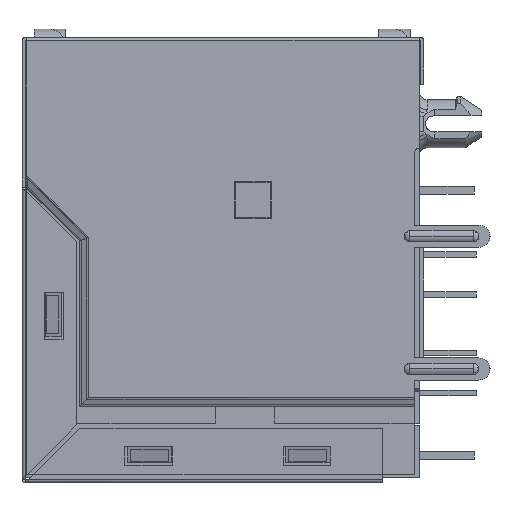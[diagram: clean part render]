
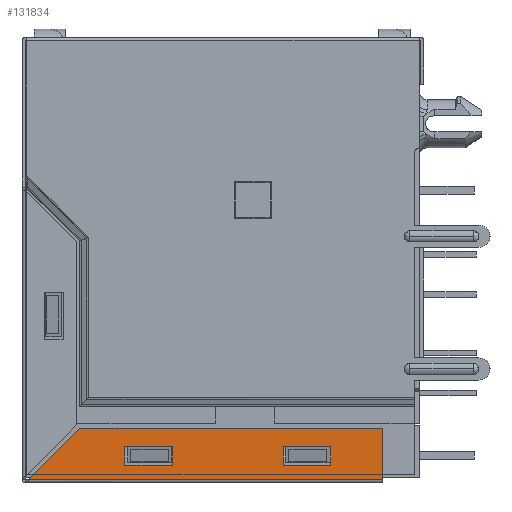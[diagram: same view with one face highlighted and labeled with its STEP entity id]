
A CAD part, left-side view. The second image highlights one B-rep face of the part: STEP entity #131834.
In plain terms, the highlighted planar face has unit normal (-1, 0, 0).
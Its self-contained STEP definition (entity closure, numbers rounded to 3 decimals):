
#479 = EDGE_CURVE ( 'NONE', #92332, #122461, #67862, .T. ) ;
#1755 = CARTESIAN_POINT ( 'NONE',  ( -31.875, -6.835, -26.78 ) ) ;
#2721 = CARTESIAN_POINT ( 'NONE',  ( -31.875, -6.835, -25.58 ) ) ;
#3954 = CARTESIAN_POINT ( 'NONE',  ( -31.875, 9.005, -24.43 ) ) ;
#6766 = CARTESIAN_POINT ( 'NONE',  ( -31.875, 9.005, -24.43 ) ) ;
#7658 = AXIS2_PLACEMENT_3D ( 'NONE', #82302, #104443, #136726 ) ;
#8901 = VERTEX_POINT ( 'NONE', #135240 ) ;
#9301 = ORIENTED_EDGE ( 'NONE', *, *, #128869, .T. ) ;
#12547 = VERTEX_POINT ( 'NONE', #30145 ) ;
#12951 = VERTEX_POINT ( 'NONE', #25709 ) ;
#13915 = EDGE_CURVE ( 'NONE', #138499, #12951, #78250, .T. ) ;
#15369 = CARTESIAN_POINT ( 'NONE',  ( -31.875, -6.835, -26.78 ) ) ;
#18320 = ORIENTED_EDGE ( 'NONE', *, *, #48286, .F. ) ;
#22806 = EDGE_CURVE ( 'NONE', #122461, #8901, #53511, .T. ) ;
#23165 = B_SPLINE_CURVE_WITH_KNOTS ( 'NONE', 1,
 ( #71344, #26937 ),
 .UNSPECIFIED., .F., .F.,
 ( 2, 2 ),
 ( 0., 1. ),
 .UNSPECIFIED. ) ;
#25709 = CARTESIAN_POINT ( 'NONE',  ( -31.875, -10.135, -24.43 ) ) ;
#26937 = CARTESIAN_POINT ( 'NONE',  ( -31.875, -10.135, -27.67 ) ) ;
#27816 = FACE_BOUND ( 'NONE', #97887, .T. ) ;
#28382 = EDGE_CURVE ( 'NONE', #57053, #57291, #94023, .T. ) ;
#30145 = CARTESIAN_POINT ( 'NONE',  ( -31.875, 3.165, -25.58 ) ) ;
#31083 = B_SPLINE_CURVE_WITH_KNOTS ( 'NONE', 1,
 ( #90847, #58183 ),
 .UNSPECIFIED., .F., .F.,
 ( 2, 2 ),
 ( 0., 1. ),
 .UNSPECIFIED. ) ;
#31956 = CARTESIAN_POINT ( 'NONE',  ( -31.875, -6.835, -25.58 ) ) ;
#37883 = CARTESIAN_POINT ( 'NONE',  ( -31.875, 12.245, -27.67 ) ) ;
#38693 = CARTESIAN_POINT ( 'NONE',  ( -31.875, 3.165, -26.78 ) ) ;
#43292 = CARTESIAN_POINT ( 'NONE',  ( -31.875, 3.165, -26.78 ) ) ;
#44898 = EDGE_CURVE ( 'NONE', #12547, #78756, #121286, .T. ) ;
#45583 = ORIENTED_EDGE ( 'NONE', *, *, #479, .T. ) ;
#47534 = CARTESIAN_POINT ( 'NONE',  ( -31.875, 3.165, -25.58 ) ) ;
#48286 = EDGE_CURVE ( 'NONE', #12951, #57291, #23165, .T. ) ;
#49384 = EDGE_LOOP ( 'NONE', ( #9301, #84357, #45583, #81935 ) ) ;
#51199 = CARTESIAN_POINT ( 'NONE',  ( -31.875, 12.245, -27.67 ) ) ;
#51403 = CARTESIAN_POINT ( 'NONE',  ( -31.875, -10.135, -24.43 ) ) ;
#53511 = B_SPLINE_CURVE_WITH_KNOTS ( 'NONE', 1,
 ( #82956, #61356 ),
 .UNSPECIFIED., .F., .F.,
 ( 2, 2 ),
 ( 0., 1. ),
 .UNSPECIFIED. ) ;
#53728 = CARTESIAN_POINT ( 'NONE',  ( -31.875, -3.835, -25.58 ) ) ;
#54936 = B_SPLINE_CURVE_WITH_KNOTS ( 'NONE', 1,
 ( #107171, #75411 ),
 .UNSPECIFIED., .F., .F.,
 ( 2, 2 ),
 ( 0., 1. ),
 .UNSPECIFIED. ) ;
#55385 = EDGE_LOOP ( 'NONE', ( #62046, #84402, #18320, #114992 ) ) ;
#56720 = CARTESIAN_POINT ( 'NONE',  ( -31.875, 6.165, -26.78 ) ) ;
#57053 = VERTEX_POINT ( 'NONE', #51199 ) ;
#57291 = VERTEX_POINT ( 'NONE', #133423 ) ;
#58183 = CARTESIAN_POINT ( 'NONE',  ( -31.875, 6.165, -25.58 ) ) ;
#60701 = EDGE_CURVE ( 'NONE', #78756, #77071, #54936, .T. ) ;
#61356 = CARTESIAN_POINT ( 'NONE',  ( -31.875, -3.835, -26.78 ) ) ;
#62046 = ORIENTED_EDGE ( 'NONE', *, *, #113118, .F. ) ;
#63472 = VERTEX_POINT ( 'NONE', #104632 ) ;
#63541 = CARTESIAN_POINT ( 'NONE',  ( -31.875, -3.835, -26.78 ) ) ;
#67862 = B_SPLINE_CURVE_WITH_KNOTS ( 'NONE', 1,
 ( #2721, #1755 ),
 .UNSPECIFIED., .F., .F.,
 ( 2, 2 ),
 ( 0., 1. ),
 .UNSPECIFIED. ) ;
#69342 = CARTESIAN_POINT ( 'NONE',  ( -31.875, 12.245, -27.67 ) ) ;
#71344 = CARTESIAN_POINT ( 'NONE',  ( -31.875, -10.135, -24.43 ) ) ;
#75209 = B_SPLINE_CURVE_WITH_KNOTS ( 'NONE', 1,
 ( #63541, #85172 ),
 .UNSPECIFIED., .F., .F.,
 ( 2, 2 ),
 ( 0., 1. ),
 .UNSPECIFIED. ) ;
#75411 = CARTESIAN_POINT ( 'NONE',  ( -31.875, 6.165, -26.78 ) ) ;
#77071 = VERTEX_POINT ( 'NONE', #56720 ) ;
#78250 = B_SPLINE_CURVE_WITH_KNOTS ( 'NONE', 1,
 ( #6766, #51403 ),
 .UNSPECIFIED., .F., .F.,
 ( 2, 2 ),
 ( 0., 1. ),
 .UNSPECIFIED. ) ;
#78756 = VERTEX_POINT ( 'NONE', #43292 ) ;
#81935 = ORIENTED_EDGE ( 'NONE', *, *, #22806, .T. ) ;
#82302 = CARTESIAN_POINT ( 'NONE',  ( -31.875, 12.693, -27.766 ) ) ;
#82956 = CARTESIAN_POINT ( 'NONE',  ( -31.875, -6.835, -26.78 ) ) ;
#84357 = ORIENTED_EDGE ( 'NONE', *, *, #120521, .T. ) ;
#84402 = ORIENTED_EDGE ( 'NONE', *, *, #28382, .T. ) ;
#84960 = B_SPLINE_CURVE_WITH_KNOTS ( 'NONE', 1,
 ( #37883, #3954 ),
 .UNSPECIFIED., .F., .F.,
 ( 2, 2 ),
 ( 0., 1. ),
 .UNSPECIFIED. ) ;
#85172 = CARTESIAN_POINT ( 'NONE',  ( -31.875, -3.835, -25.58 ) ) ;
#87568 = CARTESIAN_POINT ( 'NONE',  ( -31.875, 9.005, -24.43 ) ) ;
#90847 = CARTESIAN_POINT ( 'NONE',  ( -31.875, 6.165, -26.78 ) ) ;
#92332 = VERTEX_POINT ( 'NONE', #134268 ) ;
#94023 = B_SPLINE_CURVE_WITH_KNOTS ( 'NONE', 1,
 ( #69342, #124720 ),
 .UNSPECIFIED., .F., .F.,
 ( 2, 2 ),
 ( 0., 1. ),
 .UNSPECIFIED. ) ;
#94053 = CARTESIAN_POINT ( 'NONE',  ( -31.875, 3.165, -25.58 ) ) ;
#94308 = ORIENTED_EDGE ( 'NONE', *, *, #115554, .T. ) ;
#97887 = EDGE_LOOP ( 'NONE', ( #94308, #129240, #104714, #135754 ) ) ;
#98158 = B_SPLINE_CURVE_WITH_KNOTS ( 'NONE', 1,
 ( #135212, #47534 ),
 .UNSPECIFIED., .F., .F.,
 ( 2, 2 ),
 ( 0., 1. ),
 .UNSPECIFIED. ) ;
#104443 = DIRECTION ( 'NONE',  ( -1., 0., 0. ) ) ;
#104632 = CARTESIAN_POINT ( 'NONE',  ( -31.875, 6.165, -25.58 ) ) ;
#104714 = ORIENTED_EDGE ( 'NONE', *, *, #44898, .T. ) ;
#107171 = CARTESIAN_POINT ( 'NONE',  ( -31.875, 3.165, -26.78 ) ) ;
#110737 = FACE_BOUND ( 'NONE', #49384, .T. ) ;
#113118 = EDGE_CURVE ( 'NONE', #57053, #138499, #84960, .T. ) ;
#114992 = ORIENTED_EDGE ( 'NONE', *, *, #13915, .F. ) ;
#115554 = EDGE_CURVE ( 'NONE', #77071, #63472, #31083, .T. ) ;
#116469 = PLANE ( 'NONE',  #7658 ) ;
#117573 = B_SPLINE_CURVE_WITH_KNOTS ( 'NONE', 1,
 ( #53728, #31956 ),
 .UNSPECIFIED., .F., .F.,
 ( 2, 2 ),
 ( 0., 1. ),
 .UNSPECIFIED. ) ;
#119136 = VERTEX_POINT ( 'NONE', #141273 ) ;
#120521 = EDGE_CURVE ( 'NONE', #119136, #92332, #117573, .T. ) ;
#121286 = B_SPLINE_CURVE_WITH_KNOTS ( 'NONE', 1,
 ( #94053, #38693 ),
 .UNSPECIFIED., .F., .F.,
 ( 2, 2 ),
 ( 0., 1. ),
 .UNSPECIFIED. ) ;
#121961 = EDGE_CURVE ( 'NONE', #63472, #12547, #98158, .T. ) ;
#122461 = VERTEX_POINT ( 'NONE', #15369 ) ;
#122691 = FACE_OUTER_BOUND ( 'NONE', #55385, .T. ) ;
#124720 = CARTESIAN_POINT ( 'NONE',  ( -31.875, -10.135, -27.67 ) ) ;
#128869 = EDGE_CURVE ( 'NONE', #8901, #119136, #75209, .T. ) ;
#129240 = ORIENTED_EDGE ( 'NONE', *, *, #121961, .T. ) ;
#131834 = ADVANCED_FACE ( 'NONE', ( #122691, #27816, #110737 ), #116469, .T. ) ;
#133423 = CARTESIAN_POINT ( 'NONE',  ( -31.875, -10.135, -27.67 ) ) ;
#134268 = CARTESIAN_POINT ( 'NONE',  ( -31.875, -6.835, -25.58 ) ) ;
#135212 = CARTESIAN_POINT ( 'NONE',  ( -31.875, 6.165, -25.58 ) ) ;
#135240 = CARTESIAN_POINT ( 'NONE',  ( -31.875, -3.835, -26.78 ) ) ;
#135754 = ORIENTED_EDGE ( 'NONE', *, *, #60701, .T. ) ;
#136726 = DIRECTION ( 'NONE',  ( 0., -1., 0. ) ) ;
#138499 = VERTEX_POINT ( 'NONE', #87568 ) ;
#141273 = CARTESIAN_POINT ( 'NONE',  ( -31.875, -3.835, -25.58 ) ) ;
